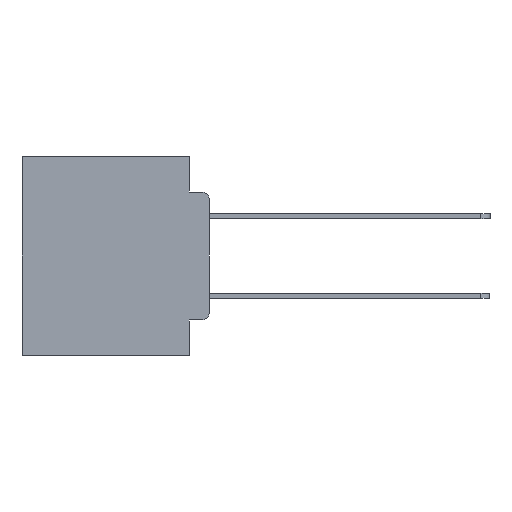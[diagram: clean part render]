
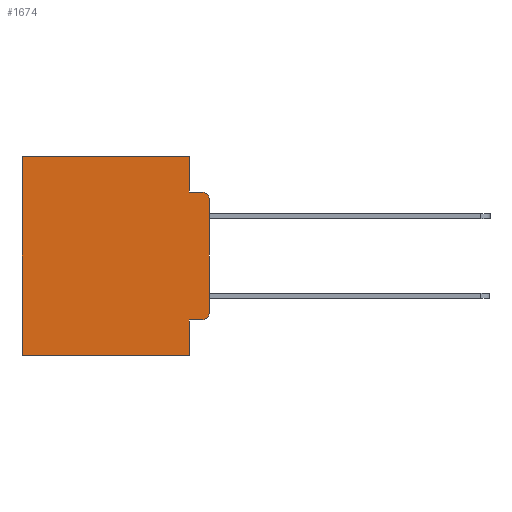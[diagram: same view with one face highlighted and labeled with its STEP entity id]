
A CAD part, left-side view. The second image highlights one B-rep face of the part: STEP entity #1674.
In plain terms, the highlighted planar face has unit normal (-1, 0, 0).
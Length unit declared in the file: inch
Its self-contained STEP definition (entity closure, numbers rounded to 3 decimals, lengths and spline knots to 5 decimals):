
#816 = DIRECTION ( 'NONE',  ( 0., 0., -1. ) ) ;
#1146 = ORIENTED_EDGE ( 'NONE', *, *, #6276, .T. ) ;
#1250 = CARTESIAN_POINT ( 'NONE',  ( 0.298, 0.02, -0.3915 ) ) ;
#1447 = EDGE_CURVE ( 'NONE', #20426, #22729, #5531, .T. ) ;
#1674 = ADVANCED_FACE ( 'NONE', ( #5851 ), #14932, .F. ) ;
#2001 = DIRECTION ( 'NONE',  ( 0., -1., 0. ) ) ;
#2008 = VERTEX_POINT ( 'NONE', #22466 ) ;
#3250 = CARTESIAN_POINT ( 'NONE',  ( 0.298, 0., -0.5 ) ) ;
#3279 = VERTEX_POINT ( 'NONE', #19369 ) ;
#3599 = DIRECTION ( 'NONE',  ( 0., 0., -1. ) ) ;
#4009 = EDGE_CURVE ( 'NONE', #6640, #11156, #22591, .T. ) ;
#4226 = CARTESIAN_POINT ( 'NONE',  ( 0.298, 0.051, -0.5 ) ) ;
#4342 = EDGE_CURVE ( 'NONE', #20574, #8341, #19565, .T. ) ;
#4777 = VECTOR ( 'NONE', #23423, 39.37008 ) ;
#5112 = LINE ( 'NONE', #20870, #16012 ) ;
#5219 = AXIS2_PLACEMENT_3D ( 'NONE', #1250, #16683, #3599 ) ;
#5531 = LINE ( 'NONE', #3250, #27708 ) ;
#5851 = FACE_OUTER_BOUND ( 'NONE', #9960, .T. ) ;
#6014 = ORIENTED_EDGE ( 'NONE', *, *, #1447, .F. ) ;
#6276 = EDGE_CURVE ( 'NONE', #14390, #16673, #12393, .T. ) ;
#6640 = VERTEX_POINT ( 'NONE', #11309 ) ;
#6645 = CARTESIAN_POINT ( 'NONE',  ( 0.298, 0.473, -0.5 ) ) ;
#6702 = VECTOR ( 'NONE', #15587, 39.37008 ) ;
#8091 = EDGE_CURVE ( 'NONE', #20574, #11156, #8922, .T. ) ;
#8341 = VERTEX_POINT ( 'NONE', #12721 ) ;
#8365 = CARTESIAN_POINT ( 'NONE',  ( 0.298, 0.02, -0.4115 ) ) ;
#8922 = CIRCLE ( 'NONE', #27619, 0.02 ) ;
#9272 = CARTESIAN_POINT ( 'NONE',  ( 0.298, 0.02, -0.0885 ) ) ;
#9811 = DIRECTION ( 'NONE',  ( 0., 0., -1. ) ) ;
#9960 = EDGE_LOOP ( 'NONE', ( #10287, #21366, #20032, #10726, #17476, #18944, #6014, #20642, #1146, #17445 ) ) ;
#10287 = ORIENTED_EDGE ( 'NONE', *, *, #4342, .F. ) ;
#10726 = ORIENTED_EDGE ( 'NONE', *, *, #25689, .F. ) ;
#10863 = CARTESIAN_POINT ( 'NONE',  ( 0.298, 0.051, -0.0885 ) ) ;
#11156 = VERTEX_POINT ( 'NONE', #9272 ) ;
#11309 = CARTESIAN_POINT ( 'NONE',  ( 0.298, 0.051, -0.0885 ) ) ;
#11768 = CARTESIAN_POINT ( 'NONE',  ( 0.298, 0., 0. ) ) ;
#12323 = DIRECTION ( 'NONE',  ( 0., 0., -1. ) ) ;
#12379 = DIRECTION ( 'NONE',  ( 0., -1., 0. ) ) ;
#12393 = LINE ( 'NONE', #25151, #18127 ) ;
#12444 = CARTESIAN_POINT ( 'NONE',  ( 0.298, 0.051, -0.4115 ) ) ;
#12721 = CARTESIAN_POINT ( 'NONE',  ( 0.298, 0., -0.3915 ) ) ;
#13813 = EDGE_CURVE ( 'NONE', #2008, #3279, #27663, .T. ) ;
#13884 = VECTOR ( 'NONE', #9811, 39.37008 ) ;
#14172 = DIRECTION ( 'NONE',  ( -1., 0., 0. ) ) ;
#14390 = VERTEX_POINT ( 'NONE', #12444 ) ;
#14659 = EDGE_CURVE ( 'NONE', #14390, #20426, #26286, .T. ) ;
#14932 = PLANE ( 'NONE',  #22601 ) ;
#14969 = VECTOR ( 'NONE', #15527, 39.37008 ) ;
#15527 = DIRECTION ( 'NONE',  ( 0., 0., -1. ) ) ;
#15587 = DIRECTION ( 'NONE',  ( 0., 0., -1. ) ) ;
#16012 = VECTOR ( 'NONE', #12323, 39.37008 ) ;
#16673 = VERTEX_POINT ( 'NONE', #8365 ) ;
#16683 = DIRECTION ( 'NONE',  ( -1., 0., 0. ) ) ;
#16881 = VECTOR ( 'NONE', #2001, 39.37008 ) ;
#17445 = ORIENTED_EDGE ( 'NONE', *, *, #20786, .T. ) ;
#17476 = ORIENTED_EDGE ( 'NONE', *, *, #13813, .T. ) ;
#17553 = LINE ( 'NONE', #19827, #6702 ) ;
#17939 = CARTESIAN_POINT ( 'NONE',  ( 0.298, 0., -0.1085 ) ) ;
#18127 = VECTOR ( 'NONE', #12379, 39.37008 ) ;
#18410 = CARTESIAN_POINT ( 'NONE',  ( 0.298, 0., 0. ) ) ;
#18944 = ORIENTED_EDGE ( 'NONE', *, *, #23774, .T. ) ;
#19369 = CARTESIAN_POINT ( 'NONE',  ( 0.298, 0.473, 0. ) ) ;
#19565 = LINE ( 'NONE', #18410, #13884 ) ;
#19827 = CARTESIAN_POINT ( 'NONE',  ( 0.298, 0.051, 0. ) ) ;
#20032 = ORIENTED_EDGE ( 'NONE', *, *, #4009, .F. ) ;
#20426 = VERTEX_POINT ( 'NONE', #4226 ) ;
#20574 = VERTEX_POINT ( 'NONE', #17939 ) ;
#20642 = ORIENTED_EDGE ( 'NONE', *, *, #14659, .F. ) ;
#20786 = EDGE_CURVE ( 'NONE', #16673, #8341, #25101, .T. ) ;
#20870 = CARTESIAN_POINT ( 'NONE',  ( 0.298, 0.473, 0. ) ) ;
#21294 = CARTESIAN_POINT ( 'NONE',  ( 0.298, 0., 0. ) ) ;
#21366 = ORIENTED_EDGE ( 'NONE', *, *, #8091, .T. ) ;
#22466 = CARTESIAN_POINT ( 'NONE',  ( 0.298, 0.051, 0. ) ) ;
#22591 = LINE ( 'NONE', #10863, #16881 ) ;
#22601 = AXIS2_PLACEMENT_3D ( 'NONE', #11768, #24176, #26958 ) ;
#22729 = VERTEX_POINT ( 'NONE', #6645 ) ;
#22826 = DIRECTION ( 'NONE',  ( 0., 1., 0. ) ) ;
#23423 = DIRECTION ( 'NONE',  ( 0., 1., 0. ) ) ;
#23774 = EDGE_CURVE ( 'NONE', #3279, #22729, #5112, .T. ) ;
#23926 = CARTESIAN_POINT ( 'NONE',  ( 0.298, 0.051, 0. ) ) ;
#24176 = DIRECTION ( 'NONE',  ( 1., 0., 0. ) ) ;
#25101 = CIRCLE ( 'NONE', #5219, 0.02 ) ;
#25151 = CARTESIAN_POINT ( 'NONE',  ( 0.298, 0.051, -0.4115 ) ) ;
#25689 = EDGE_CURVE ( 'NONE', #2008, #6640, #17553, .T. ) ;
#26286 = LINE ( 'NONE', #23926, #14969 ) ;
#26884 = CARTESIAN_POINT ( 'NONE',  ( 0.298, 0.02, -0.1085 ) ) ;
#26958 = DIRECTION ( 'NONE',  ( 0., 0., -1. ) ) ;
#27619 = AXIS2_PLACEMENT_3D ( 'NONE', #26884, #14172, #816 ) ;
#27663 = LINE ( 'NONE', #21294, #4777 ) ;
#27708 = VECTOR ( 'NONE', #22826, 39.37008 ) ;
